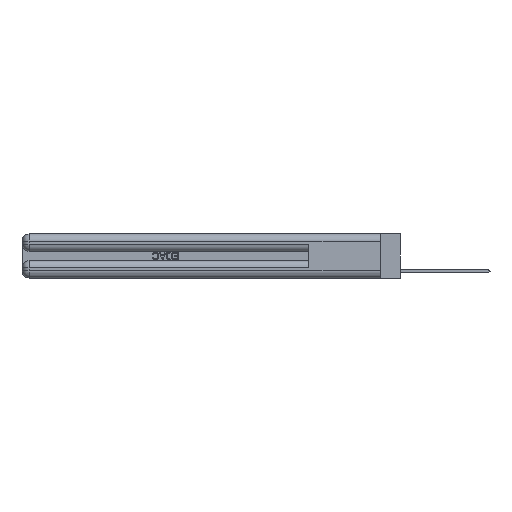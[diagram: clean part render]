
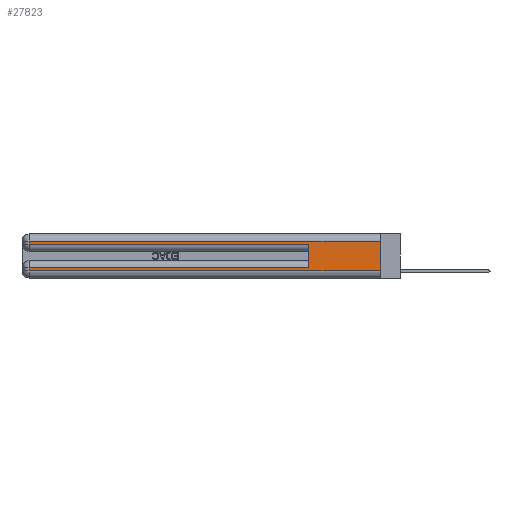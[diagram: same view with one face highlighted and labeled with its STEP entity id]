
A CAD part, left-side view. The second image highlights one B-rep face of the part: STEP entity #27823.
In plain terms, the highlighted planar face has unit normal (-1, 0, 0).
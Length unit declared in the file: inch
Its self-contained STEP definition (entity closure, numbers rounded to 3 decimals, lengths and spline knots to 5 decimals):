
#403 = ORIENTED_EDGE ( 'NONE', *, *, #7638, .T. ) ;
#1107 = DIRECTION ( 'NONE',  ( 1., 0., 0. ) ) ;
#1619 = LINE ( 'NONE', #26381, #23721 ) ;
#1943 = VERTEX_POINT ( 'NONE', #27909 ) ;
#2226 = LINE ( 'NONE', #14962, #4447 ) ;
#3182 = FACE_OUTER_BOUND ( 'NONE', #9218, .T. ) ;
#3209 = VECTOR ( 'NONE', #11712, 39.37008 ) ;
#4269 = EDGE_CURVE ( 'NONE', #6907, #14318, #21784, .T. ) ;
#4280 = ORIENTED_EDGE ( 'NONE', *, *, #12716, .F. ) ;
#4311 = AXIS2_PLACEMENT_3D ( 'NONE', #26303, #1107, #17101 ) ;
#4351 = LINE ( 'NONE', #15507, #20630 ) ;
#4447 = VECTOR ( 'NONE', #19762, 39.37008 ) ;
#4671 = EDGE_CURVE ( 'NONE', #10360, #11635, #2226, .T. ) ;
#5024 = CARTESIAN_POINT ( 'NONE',  ( 0., 0., 0.31 ) ) ;
#5232 = LINE ( 'NONE', #25914, #26981 ) ;
#5251 = LINE ( 'NONE', #6143, #29160 ) ;
#5734 = VERTEX_POINT ( 'NONE', #9180 ) ;
#6143 = CARTESIAN_POINT ( 'NONE',  ( 0., 2.94, 0.37 ) ) ;
#6901 = VERTEX_POINT ( 'NONE', #25904 ) ;
#6907 = VERTEX_POINT ( 'NONE', #5024 ) ;
#7638 = EDGE_CURVE ( 'NONE', #11635, #9990, #15497, .T. ) ;
#8356 = CARTESIAN_POINT ( 'NONE',  ( 0., 2.94, 0.31 ) ) ;
#8583 = EDGE_CURVE ( 'NONE', #14318, #5734, #5251, .T. ) ;
#9180 = CARTESIAN_POINT ( 'NONE',  ( 0., 2.94, 0.285 ) ) ;
#9218 = EDGE_LOOP ( 'NONE', ( #22987, #12827, #28637, #22011, #4280, #11451, #24898, #403 ) ) ;
#9990 = VERTEX_POINT ( 'NONE', #15002 ) ;
#10360 = VERTEX_POINT ( 'NONE', #19324 ) ;
#10625 = DIRECTION ( 'NONE',  ( 0., 0., -1. ) ) ;
#11451 = ORIENTED_EDGE ( 'NONE', *, *, #20694, .T. ) ;
#11635 = VERTEX_POINT ( 'NONE', #21718 ) ;
#11712 = DIRECTION ( 'NONE',  ( 0., -1., 0. ) ) ;
#12716 = EDGE_CURVE ( 'NONE', #6901, #1943, #5232, .T. ) ;
#12827 = ORIENTED_EDGE ( 'NONE', *, *, #4269, .T. ) ;
#12846 = PLANE ( 'NONE',  #4311 ) ;
#13786 = VECTOR ( 'NONE', #27541, 39.37008 ) ;
#14184 = VECTOR ( 'NONE', #23498, 39.37008 ) ;
#14318 = VERTEX_POINT ( 'NONE', #8356 ) ;
#14962 = CARTESIAN_POINT ( 'NONE',  ( 0., 2.94, 0.37 ) ) ;
#15002 = CARTESIAN_POINT ( 'NONE',  ( 0., 0., 0.06 ) ) ;
#15497 = LINE ( 'NONE', #25581, #3209 ) ;
#15507 = CARTESIAN_POINT ( 'NONE',  ( 0., 0., 0.37 ) ) ;
#15722 = CARTESIAN_POINT ( 'NONE',  ( 0., 0., 0.285 ) ) ;
#17101 = DIRECTION ( 'NONE',  ( 0., 0., -1. ) ) ;
#19068 = DIRECTION ( 'NONE',  ( 0., 0., 1. ) ) ;
#19324 = CARTESIAN_POINT ( 'NONE',  ( 0., 2.94, 0.085 ) ) ;
#19762 = DIRECTION ( 'NONE',  ( 0., 0., -1. ) ) ;
#20630 = VECTOR ( 'NONE', #27423, 39.37008 ) ;
#20694 = EDGE_CURVE ( 'NONE', #6901, #10360, #1619, .T. ) ;
#20696 = DIRECTION ( 'NONE',  ( 0., 1., 0. ) ) ;
#21452 = CARTESIAN_POINT ( 'NONE',  ( 0., 0., 0.31 ) ) ;
#21718 = CARTESIAN_POINT ( 'NONE',  ( 0., 2.94, 0.06 ) ) ;
#21784 = LINE ( 'NONE', #21452, #14184 ) ;
#22011 = ORIENTED_EDGE ( 'NONE', *, *, #26091, .T. ) ;
#22987 = ORIENTED_EDGE ( 'NONE', *, *, #26763, .F. ) ;
#23208 = LINE ( 'NONE', #15722, #13786 ) ;
#23498 = DIRECTION ( 'NONE',  ( 0., 1., 0. ) ) ;
#23721 = VECTOR ( 'NONE', #20696, 39.37008 ) ;
#24898 = ORIENTED_EDGE ( 'NONE', *, *, #4671, .T. ) ;
#25581 = CARTESIAN_POINT ( 'NONE',  ( 0., 0., 0.06 ) ) ;
#25904 = CARTESIAN_POINT ( 'NONE',  ( 0., 0.6, 0.085 ) ) ;
#25914 = CARTESIAN_POINT ( 'NONE',  ( 0., 0.6, 0.145 ) ) ;
#26091 = EDGE_CURVE ( 'NONE', #5734, #1943, #23208, .T. ) ;
#26303 = CARTESIAN_POINT ( 'NONE',  ( 0., 0., 0.37 ) ) ;
#26381 = CARTESIAN_POINT ( 'NONE',  ( 0., 0., 0.085 ) ) ;
#26763 = EDGE_CURVE ( 'NONE', #6907, #9990, #4351, .T. ) ;
#26981 = VECTOR ( 'NONE', #19068, 39.37008 ) ;
#27423 = DIRECTION ( 'NONE',  ( 0., 0., -1. ) ) ;
#27541 = DIRECTION ( 'NONE',  ( 0., -1., 0. ) ) ;
#27823 = ADVANCED_FACE ( 'NONE', ( #3182 ), #12846, .F. ) ;
#27909 = CARTESIAN_POINT ( 'NONE',  ( 0., 0.6, 0.285 ) ) ;
#28637 = ORIENTED_EDGE ( 'NONE', *, *, #8583, .T. ) ;
#29160 = VECTOR ( 'NONE', #10625, 39.37008 ) ;
